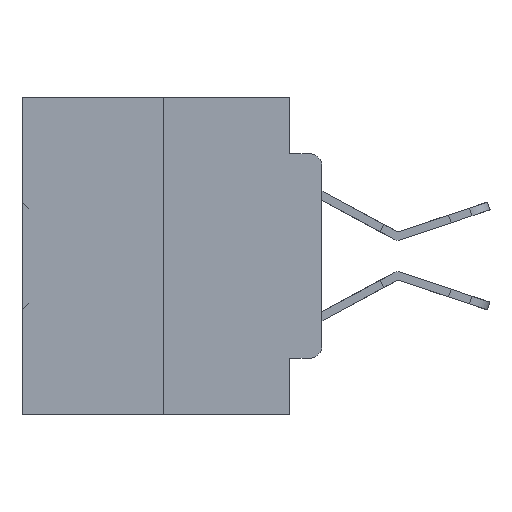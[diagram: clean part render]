
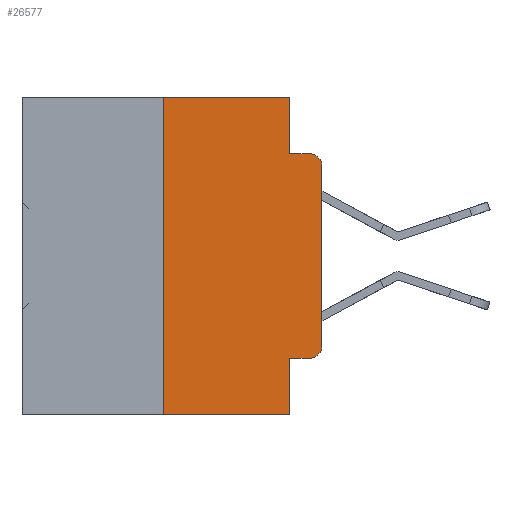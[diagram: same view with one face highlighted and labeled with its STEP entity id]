
A CAD part, left-side view. The second image highlights one B-rep face of the part: STEP entity #26577.
In plain terms, the highlighted planar face has unit normal (-1, 0, 0).
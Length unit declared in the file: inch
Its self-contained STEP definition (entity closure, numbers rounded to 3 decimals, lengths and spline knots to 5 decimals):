
#186 = ORIENTED_EDGE ( 'NONE', *, *, #14728, .F. ) ;
#931 = CIRCLE ( 'NONE', #17662, 0.02 ) ;
#952 = EDGE_CURVE ( 'NONE', #31574, #27443, #11058, .T. ) ;
#1742 = LINE ( 'NONE', #26727, #6418 ) ;
#2182 = CARTESIAN_POINT ( 'NONE',  ( 0., 0.02, -0.0885 ) ) ;
#2216 = ORIENTED_EDGE ( 'NONE', *, *, #35347, .F. ) ;
#2469 = EDGE_CURVE ( 'NONE', #33402, #31574, #31468, .T. ) ;
#2778 = CARTESIAN_POINT ( 'NONE',  ( 0., 0.051, 0. ) ) ;
#2881 = LINE ( 'NONE', #36582, #24991 ) ;
#3781 = ORIENTED_EDGE ( 'NONE', *, *, #5800, .T. ) ;
#4986 = VERTEX_POINT ( 'NONE', #30760 ) ;
#5154 = CARTESIAN_POINT ( 'NONE',  ( 0., 0.473, 0. ) ) ;
#5250 = DIRECTION ( 'NONE',  ( 0., 0., 1. ) ) ;
#5800 = EDGE_CURVE ( 'NONE', #6858, #4986, #931, .T. ) ;
#6286 = VECTOR ( 'NONE', #26928, 39.37008 ) ;
#6418 = VECTOR ( 'NONE', #13827, 39.37008 ) ;
#6828 = LINE ( 'NONE', #19127, #33992 ) ;
#6856 = CARTESIAN_POINT ( 'NONE',  ( 0., 0.051, 0. ) ) ;
#6858 = VERTEX_POINT ( 'NONE', #9379 ) ;
#7584 = FACE_OUTER_BOUND ( 'NONE', #22463, .T. ) ;
#7771 = EDGE_CURVE ( 'NONE', #33005, #10761, #6828, .T. ) ;
#8737 = CARTESIAN_POINT ( 'NONE',  ( 0., 0.25, 0. ) ) ;
#8915 = DIRECTION ( 'NONE',  ( 0., -1., 0. ) ) ;
#9379 = CARTESIAN_POINT ( 'NONE',  ( 0., 0.02, -0.4115 ) ) ;
#9962 = VECTOR ( 'NONE', #5250, 39.37008 ) ;
#10761 = VERTEX_POINT ( 'NONE', #31580 ) ;
#10793 = DIRECTION ( 'NONE',  ( -1., 0., 0. ) ) ;
#10859 = CARTESIAN_POINT ( 'NONE',  ( 0., 0., -0.1085 ) ) ;
#10989 = CARTESIAN_POINT ( 'NONE',  ( 0., 0.02, -0.1085 ) ) ;
#11058 = LINE ( 'NONE', #26979, #11246 ) ;
#11246 = VECTOR ( 'NONE', #11451, 39.37008 ) ;
#11451 = DIRECTION ( 'NONE',  ( 0., -1., 0. ) ) ;
#11560 = AXIS2_PLACEMENT_3D ( 'NONE', #5154, #32198, #17454 ) ;
#11684 = CARTESIAN_POINT ( 'NONE',  ( 0., 0.051, -0.4115 ) ) ;
#13505 = ORIENTED_EDGE ( 'NONE', *, *, #7771, .T. ) ;
#13827 = DIRECTION ( 'NONE',  ( 0., -1., 0. ) ) ;
#13862 = EDGE_CURVE ( 'NONE', #34169, #10761, #33450, .T. ) ;
#14259 = EDGE_CURVE ( 'NONE', #4986, #15072, #33205, .T. ) ;
#14309 = LINE ( 'NONE', #32882, #9962 ) ;
#14543 = AXIS2_PLACEMENT_3D ( 'NONE', #10989, #10793, #25726 ) ;
#14728 = EDGE_CURVE ( 'NONE', #25128, #33402, #2881, .T. ) ;
#14867 = DIRECTION ( 'NONE',  ( 0., 0., -1. ) ) ;
#15072 = VERTEX_POINT ( 'NONE', #10859 ) ;
#15391 = CARTESIAN_POINT ( 'NONE',  ( 0., 0.25, -0.5 ) ) ;
#17454 = DIRECTION ( 'NONE',  ( 0., 0., -1. ) ) ;
#17582 = DIRECTION ( 'NONE',  ( -1., 0., 0. ) ) ;
#17662 = AXIS2_PLACEMENT_3D ( 'NONE', #32917, #17582, #35948 ) ;
#18768 = ORIENTED_EDGE ( 'NONE', *, *, #2469, .F. ) ;
#19127 = CARTESIAN_POINT ( 'NONE',  ( 0., 0.473, -0.5 ) ) ;
#21073 = VECTOR ( 'NONE', #14867, 39.37008 ) ;
#21581 = ORIENTED_EDGE ( 'NONE', *, *, #14259, .T. ) ;
#21986 = DIRECTION ( 'NONE',  ( 0., 0., -1. ) ) ;
#22037 = ORIENTED_EDGE ( 'NONE', *, *, #952, .F. ) ;
#22463 = EDGE_LOOP ( 'NONE', ( #21581, #31029, #22037, #18768, #186, #2216, #13505, #38577, #37749, #3781 ) ) ;
#23486 = PLANE ( 'NONE',  #11560 ) ;
#23819 = CARTESIAN_POINT ( 'NONE',  ( 0., 0.051, 0. ) ) ;
#24991 = VECTOR ( 'NONE', #8915, 39.37008 ) ;
#25128 = VERTEX_POINT ( 'NONE', #8737 ) ;
#25726 = DIRECTION ( 'NONE',  ( 0., 0., -1. ) ) ;
#26577 = ADVANCED_FACE ( 'NONE', ( #7584 ), #23486, .F. ) ;
#26727 = CARTESIAN_POINT ( 'NONE',  ( 0., 0.051, -0.4115 ) ) ;
#26928 = DIRECTION ( 'NONE',  ( 0., 0., 1. ) ) ;
#26979 = CARTESIAN_POINT ( 'NONE',  ( 0., 0.051, -0.0885 ) ) ;
#27443 = VERTEX_POINT ( 'NONE', #2182 ) ;
#27977 = EDGE_CURVE ( 'NONE', #34169, #6858, #1742, .T. ) ;
#28475 = VECTOR ( 'NONE', #21986, 39.37008 ) ;
#29960 = CARTESIAN_POINT ( 'NONE',  ( 0., 0., 0. ) ) ;
#30760 = CARTESIAN_POINT ( 'NONE',  ( 0., 0., -0.3915 ) ) ;
#31029 = ORIENTED_EDGE ( 'NONE', *, *, #36048, .T. ) ;
#31468 = LINE ( 'NONE', #6856, #28475 ) ;
#31574 = VERTEX_POINT ( 'NONE', #32966 ) ;
#31580 = CARTESIAN_POINT ( 'NONE',  ( 0., 0.051, -0.5 ) ) ;
#31639 = DIRECTION ( 'NONE',  ( 0., -1., 0. ) ) ;
#32198 = DIRECTION ( 'NONE',  ( 1., 0., 0. ) ) ;
#32882 = CARTESIAN_POINT ( 'NONE',  ( 0., 0.25, 0. ) ) ;
#32917 = CARTESIAN_POINT ( 'NONE',  ( 0., 0.02, -0.3915 ) ) ;
#32966 = CARTESIAN_POINT ( 'NONE',  ( 0., 0.051, -0.0885 ) ) ;
#33005 = VERTEX_POINT ( 'NONE', #15391 ) ;
#33205 = LINE ( 'NONE', #29960, #6286 ) ;
#33402 = VERTEX_POINT ( 'NONE', #23819 ) ;
#33450 = LINE ( 'NONE', #2778, #21073 ) ;
#33992 = VECTOR ( 'NONE', #31639, 39.37008 ) ;
#34169 = VERTEX_POINT ( 'NONE', #11684 ) ;
#35179 = CIRCLE ( 'NONE', #14543, 0.02 ) ;
#35347 = EDGE_CURVE ( 'NONE', #33005, #25128, #14309, .T. ) ;
#35948 = DIRECTION ( 'NONE',  ( 0., 0., -1. ) ) ;
#36048 = EDGE_CURVE ( 'NONE', #15072, #27443, #35179, .T. ) ;
#36582 = CARTESIAN_POINT ( 'NONE',  ( 0., 0.473, 0. ) ) ;
#37749 = ORIENTED_EDGE ( 'NONE', *, *, #27977, .T. ) ;
#38577 = ORIENTED_EDGE ( 'NONE', *, *, #13862, .F. ) ;
